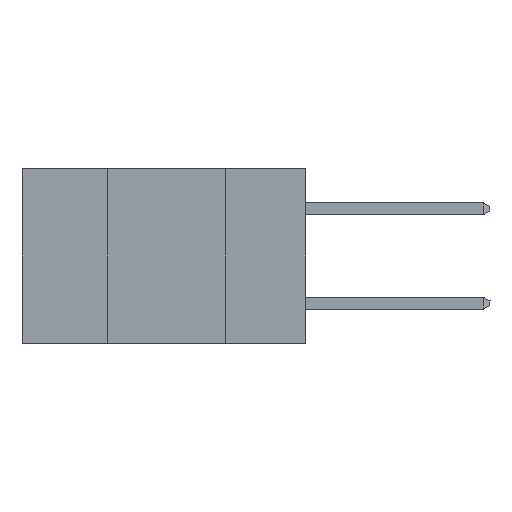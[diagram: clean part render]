
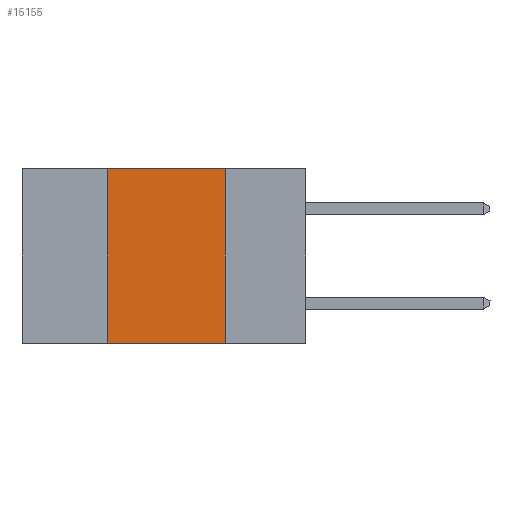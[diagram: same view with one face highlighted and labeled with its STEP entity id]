
A CAD part, left-side view. The second image highlights one B-rep face of the part: STEP entity #15155.
In plain terms, the highlighted planar face has unit normal (-1, 0, 0).
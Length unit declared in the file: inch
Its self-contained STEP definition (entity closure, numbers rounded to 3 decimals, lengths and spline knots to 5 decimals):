
#427 = ORIENTED_EDGE ( 'NONE', *, *, #10303, .T. ) ;
#1291 = VERTEX_POINT ( 'NONE', #17309 ) ;
#1394 = VERTEX_POINT ( 'NONE', #17091 ) ;
#1433 = CARTESIAN_POINT ( 'NONE',  ( 0., 0.42, 0. ) ) ;
#1440 = DIRECTION ( 'NONE',  ( 0., 0., -1. ) ) ;
#1859 = ORIENTED_EDGE ( 'NONE', *, *, #22142, .F. ) ;
#2283 = DIRECTION ( 'NONE',  ( 0., 0., -1. ) ) ;
#2293 = VECTOR ( 'NONE', #10595, 39.37008 ) ;
#2636 = LINE ( 'NONE', #19104, #7899 ) ;
#3079 = DIRECTION ( 'NONE',  ( 0., -1., 0. ) ) ;
#3865 = EDGE_CURVE ( 'NONE', #1291, #8712, #2636, .T. ) ;
#3940 = VECTOR ( 'NONE', #22366, 39.37008 ) ;
#4575 = CARTESIAN_POINT ( 'NONE',  ( 0., 0.6, 0. ) ) ;
#5967 = FACE_OUTER_BOUND ( 'NONE', #11723, .T. ) ;
#6716 = ORIENTED_EDGE ( 'NONE', *, *, #18661, .F. ) ;
#7899 = VECTOR ( 'NONE', #1440, 39.37008 ) ;
#8559 = LINE ( 'NONE', #24874, #15316 ) ;
#8712 = VERTEX_POINT ( 'NONE', #19962 ) ;
#9108 = VERTEX_POINT ( 'NONE', #1433 ) ;
#9177 = LINE ( 'NONE', #4575, #3940 ) ;
#10303 = EDGE_CURVE ( 'NONE', #1394, #8712, #8559, .T. ) ;
#10595 = DIRECTION ( 'NONE',  ( 0., 0., 1. ) ) ;
#11438 = AXIS2_PLACEMENT_3D ( 'NONE', #16187, #17952, #2283 ) ;
#11723 = EDGE_LOOP ( 'NONE', ( #16763, #6716, #1859, #427 ) ) ;
#14536 = CARTESIAN_POINT ( 'NONE',  ( 0., 0.42, 0. ) ) ;
#15155 = ADVANCED_FACE ( 'NONE', ( #5967 ), #23915, .F. ) ;
#15316 = VECTOR ( 'NONE', #3079, 39.37008 ) ;
#16187 = CARTESIAN_POINT ( 'NONE',  ( 0., 0.6, 0. ) ) ;
#16763 = ORIENTED_EDGE ( 'NONE', *, *, #3865, .F. ) ;
#17091 = CARTESIAN_POINT ( 'NONE',  ( 0., 0.42, -0.37 ) ) ;
#17309 = CARTESIAN_POINT ( 'NONE',  ( 0., 0.17, 0. ) ) ;
#17952 = DIRECTION ( 'NONE',  ( 1., 0., 0. ) ) ;
#18661 = EDGE_CURVE ( 'NONE', #9108, #1291, #9177, .T. ) ;
#19104 = CARTESIAN_POINT ( 'NONE',  ( 0., 0.17, 0. ) ) ;
#19962 = CARTESIAN_POINT ( 'NONE',  ( 0., 0.17, -0.37 ) ) ;
#22142 = EDGE_CURVE ( 'NONE', #1394, #9108, #22662, .T. ) ;
#22366 = DIRECTION ( 'NONE',  ( 0., -1., 0. ) ) ;
#22662 = LINE ( 'NONE', #14536, #2293 ) ;
#23915 = PLANE ( 'NONE',  #11438 ) ;
#24874 = CARTESIAN_POINT ( 'NONE',  ( 0., 0.6, -0.37 ) ) ;
